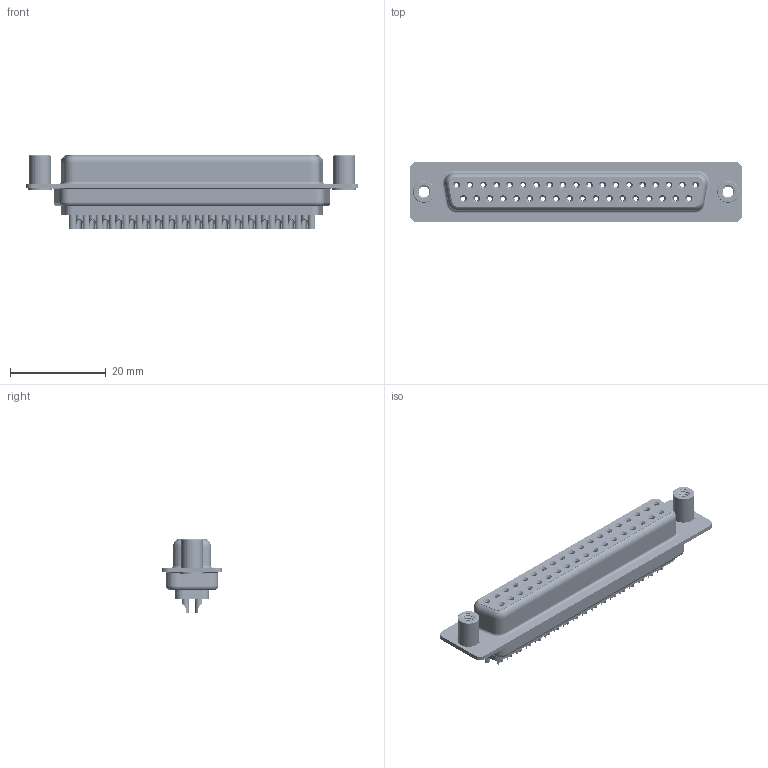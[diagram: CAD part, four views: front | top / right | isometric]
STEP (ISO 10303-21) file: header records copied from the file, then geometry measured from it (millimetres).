
FILE_DESCRIPTION (( 'STEP AP203' ), '1' );
FILE_NAME ('628-037-622-268.STEP', '2020-07-14T21:07:52', ( '' ), ( '' ), 'SwSTEP 2.0', 'SolidWorks 2020', '' );
FILE_SCHEMA (( 'CONFIG_CONTROL_DESIGN' ));
Length unit declared in the file: millimetre
Products named in the file (7): 628 Housing_37 LP; 628 Contact Row 1_22L; 628-037-622-268; 628 Shell Rear_37 Contacts; 628 Shell Front_37 Contacts; 628 Contact Row 2_22L; 628 4-40 Threaded Standoff
Assembly tree (42 placements, depth 2):
  628-037-622-268
    628 Housing_37 LP
    628 Shell Front_37 Contacts
    628 Shell Rear_37 Contacts
    628 Contact Row 1_22L  x19
    628 Contact Row 2_22L  x18
    628 4-40 Threaded Standoff  x2
Bounding box: 69.3 x 12.6 x 15.35 mm (x, y, z)
Volume: 5455.5 mm3; surface area: 13214.1 mm2
Topology: 42 solids, 42 shells, 3606 faces, 9141 edges, 5743 vertices
Faces by surface type: cylinder 1090, plane 846, bspline 746, torus 729, cone 195
Entity records: 30956 total; most frequent: CARTESIAN_POINT 8228, DIRECTION 4707, ORIENTED_EDGE 4166, EDGE_CURVE 2083, AXIS2_PLACEMENT_3D 1983, VERTEX_POINT 1320, EDGE_LOOP 1105, CIRCLE 1085
